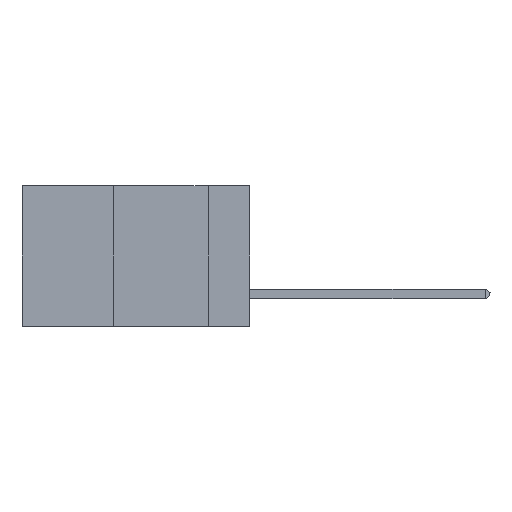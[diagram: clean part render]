
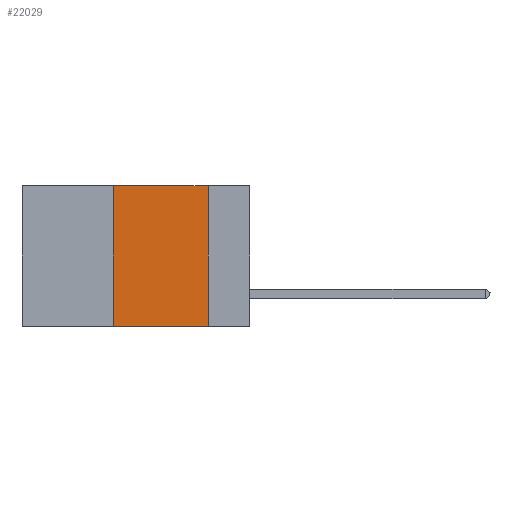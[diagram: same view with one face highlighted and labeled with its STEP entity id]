
A CAD part, left-side view. The second image highlights one B-rep face of the part: STEP entity #22029.
In plain terms, the highlighted planar face has unit normal (-1, 0, 0).
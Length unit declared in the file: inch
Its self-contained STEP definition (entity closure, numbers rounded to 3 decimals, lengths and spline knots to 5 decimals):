
#86 = VERTEX_POINT ( 'NONE', #25329 ) ;
#2201 = EDGE_CURVE ( 'NONE', #86, #12754, #27379, .T. ) ;
#2523 = ORIENTED_EDGE ( 'NONE', *, *, #4613, .T. ) ;
#3770 = LINE ( 'NONE', #13119, #39824 ) ;
#3882 = DIRECTION ( 'NONE',  ( 0., 0., -1. ) ) ;
#4613 = EDGE_CURVE ( 'NONE', #6844, #18186, #26619, .T. ) ;
#4946 = EDGE_CURVE ( 'NONE', #12754, #18186, #3770, .T. ) ;
#5039 = DIRECTION ( 'NONE',  ( 0., 0., -1. ) ) ;
#6844 = VERTEX_POINT ( 'NONE', #28137 ) ;
#8901 = CARTESIAN_POINT ( 'NONE',  ( 0., 0.11, -0.37 ) ) ;
#10932 = ORIENTED_EDGE ( 'NONE', *, *, #40050, .F. ) ;
#11047 = PLANE ( 'NONE',  #39037 ) ;
#11173 = DIRECTION ( 'NONE',  ( 0., -1., 0. ) ) ;
#11742 = ORIENTED_EDGE ( 'NONE', *, *, #2201, .F. ) ;
#12155 = LINE ( 'NONE', #37466, #35041 ) ;
#12754 = VERTEX_POINT ( 'NONE', #24835 ) ;
#13119 = CARTESIAN_POINT ( 'NONE',  ( 0., 0.11, 0. ) ) ;
#18186 = VERTEX_POINT ( 'NONE', #8901 ) ;
#19144 = VECTOR ( 'NONE', #11173, 39.37008 ) ;
#20283 = CARTESIAN_POINT ( 'NONE',  ( 0., 0.6, 0. ) ) ;
#22029 = ADVANCED_FACE ( 'NONE', ( #36686 ), #11047, .F. ) ;
#24835 = CARTESIAN_POINT ( 'NONE',  ( 0., 0.11, 0. ) ) ;
#25132 = VECTOR ( 'NONE', #36940, 39.37008 ) ;
#25329 = CARTESIAN_POINT ( 'NONE',  ( 0., 0.36, 0. ) ) ;
#25630 = ORIENTED_EDGE ( 'NONE', *, *, #4946, .F. ) ;
#26619 = LINE ( 'NONE', #34346, #25132 ) ;
#27151 = EDGE_LOOP ( 'NONE', ( #25630, #11742, #10932, #2523 ) ) ;
#27379 = LINE ( 'NONE', #32761, #19144 ) ;
#28137 = CARTESIAN_POINT ( 'NONE',  ( 0., 0.36, -0.37 ) ) ;
#32761 = CARTESIAN_POINT ( 'NONE',  ( 0., 0.6, 0. ) ) ;
#34346 = CARTESIAN_POINT ( 'NONE',  ( 0., 0.6, -0.37 ) ) ;
#35041 = VECTOR ( 'NONE', #37889, 39.37008 ) ;
#36686 = FACE_OUTER_BOUND ( 'NONE', #27151, .T. ) ;
#36940 = DIRECTION ( 'NONE',  ( 0., -1., 0. ) ) ;
#37466 = CARTESIAN_POINT ( 'NONE',  ( 0., 0.36, 0. ) ) ;
#37889 = DIRECTION ( 'NONE',  ( 0., 0., 1. ) ) ;
#39037 = AXIS2_PLACEMENT_3D ( 'NONE', #20283, #39485, #5039 ) ;
#39485 = DIRECTION ( 'NONE',  ( 1., 0., 0. ) ) ;
#39824 = VECTOR ( 'NONE', #3882, 39.37008 ) ;
#40050 = EDGE_CURVE ( 'NONE', #6844, #86, #12155, .T. ) ;
